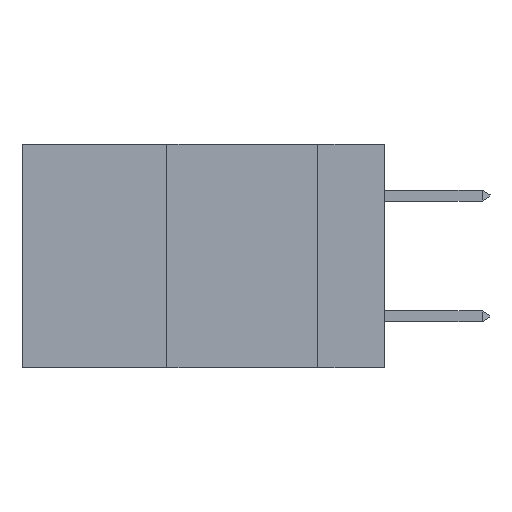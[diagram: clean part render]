
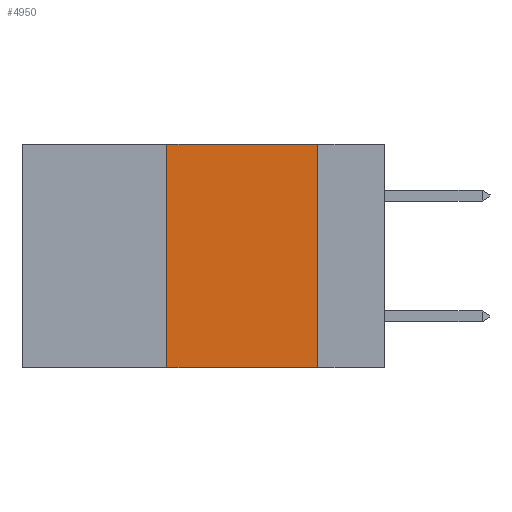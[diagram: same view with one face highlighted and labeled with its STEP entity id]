
A CAD part, left-side view. The second image highlights one B-rep face of the part: STEP entity #4950.
In plain terms, the highlighted planar face has unit normal (-1, 0, 0).
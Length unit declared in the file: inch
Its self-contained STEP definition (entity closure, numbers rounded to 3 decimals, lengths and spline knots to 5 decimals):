
#307 = LINE ( 'NONE', #3308, #5366 ) ;
#896 = CARTESIAN_POINT ( 'NONE',  ( 0., 0.6, 0. ) ) ;
#1046 = ORIENTED_EDGE ( 'NONE', *, *, #13257, .F. ) ;
#1952 = CARTESIAN_POINT ( 'NONE',  ( 0., 0.11, 0. ) ) ;
#1979 = VECTOR ( 'NONE', #10655, 39.37008 ) ;
#1981 = VERTEX_POINT ( 'NONE', #6370 ) ;
#3308 = CARTESIAN_POINT ( 'NONE',  ( 0., 0.36, 0. ) ) ;
#3320 = EDGE_CURVE ( 'NONE', #12298, #11777, #5787, .T. ) ;
#3625 = DIRECTION ( 'NONE',  ( 0., 0., -1. ) ) ;
#3660 = EDGE_CURVE ( 'NONE', #8499, #12298, #6947, .T. ) ;
#3749 = CARTESIAN_POINT ( 'NONE',  ( 0., 0.36, 0. ) ) ;
#4671 = AXIS2_PLACEMENT_3D ( 'NONE', #896, #10494, #7374 ) ;
#4950 = ADVANCED_FACE ( 'NONE', ( #5757 ), #5108, .F. ) ;
#5036 = EDGE_LOOP ( 'NONE', ( #12873, #11779, #1046, #7225 ) ) ;
#5108 = PLANE ( 'NONE',  #4671 ) ;
#5366 = VECTOR ( 'NONE', #9517, 39.37008 ) ;
#5757 = FACE_OUTER_BOUND ( 'NONE', #5036, .T. ) ;
#5787 = LINE ( 'NONE', #10114, #10556 ) ;
#5885 = CARTESIAN_POINT ( 'NONE',  ( 0., 0.6, 0. ) ) ;
#5925 = CARTESIAN_POINT ( 'NONE',  ( 0., 0.6, -0.37 ) ) ;
#6370 = CARTESIAN_POINT ( 'NONE',  ( 0., 0.36, -0.37 ) ) ;
#6947 = LINE ( 'NONE', #5885, #7609 ) ;
#7019 = CARTESIAN_POINT ( 'NONE',  ( 0., 0.11, -0.37 ) ) ;
#7225 = ORIENTED_EDGE ( 'NONE', *, *, #11176, .T. ) ;
#7374 = DIRECTION ( 'NONE',  ( 0., 0., -1. ) ) ;
#7593 = LINE ( 'NONE', #5925, #1979 ) ;
#7609 = VECTOR ( 'NONE', #10054, 39.37008 ) ;
#8499 = VERTEX_POINT ( 'NONE', #3749 ) ;
#9517 = DIRECTION ( 'NONE',  ( 0., 0., 1. ) ) ;
#10054 = DIRECTION ( 'NONE',  ( 0., -1., 0. ) ) ;
#10114 = CARTESIAN_POINT ( 'NONE',  ( 0., 0.11, 0. ) ) ;
#10494 = DIRECTION ( 'NONE',  ( 1., 0., 0. ) ) ;
#10556 = VECTOR ( 'NONE', #3625, 39.37008 ) ;
#10655 = DIRECTION ( 'NONE',  ( 0., -1., 0. ) ) ;
#11176 = EDGE_CURVE ( 'NONE', #1981, #11777, #7593, .T. ) ;
#11777 = VERTEX_POINT ( 'NONE', #7019 ) ;
#11779 = ORIENTED_EDGE ( 'NONE', *, *, #3660, .F. ) ;
#12298 = VERTEX_POINT ( 'NONE', #1952 ) ;
#12873 = ORIENTED_EDGE ( 'NONE', *, *, #3320, .F. ) ;
#13257 = EDGE_CURVE ( 'NONE', #1981, #8499, #307, .T. ) ;
